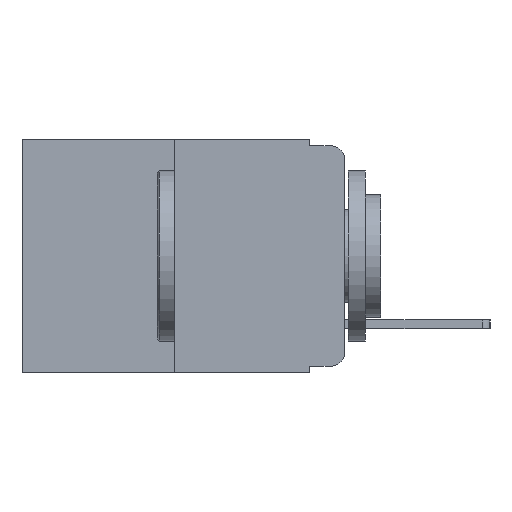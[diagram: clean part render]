
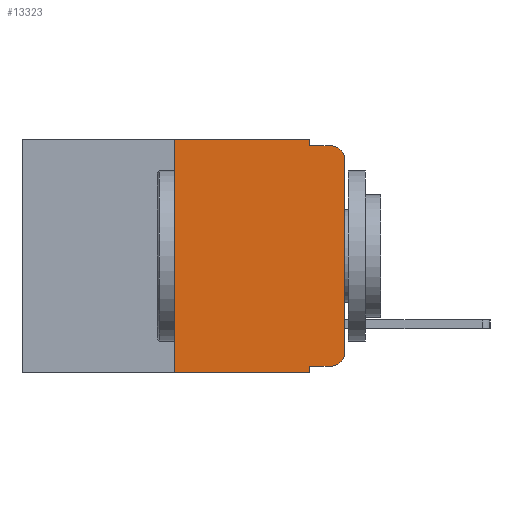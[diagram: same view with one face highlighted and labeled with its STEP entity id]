
A CAD part, left-side view. The second image highlights one B-rep face of the part: STEP entity #13323.
In plain terms, the highlighted planar face has unit normal (-1, 0, 0).
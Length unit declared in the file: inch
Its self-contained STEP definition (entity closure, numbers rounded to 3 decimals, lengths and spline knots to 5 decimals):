
#32 = VERTEX_POINT ( 'NONE', #4022 ) ;
#274 = EDGE_CURVE ( 'NONE', #12180, #11249, #820, .T. ) ;
#820 = CIRCLE ( 'NONE', #3981, 0.02 ) ;
#865 = DIRECTION ( 'NONE',  ( 0., 0., -1. ) ) ;
#1015 = DIRECTION ( 'NONE',  ( 0., 0., 1. ) ) ;
#1086 = CARTESIAN_POINT ( 'NONE',  ( 0., 0., -0.03 ) ) ;
#1105 = DIRECTION ( 'NONE',  ( 1., 0., 0. ) ) ;
#1246 = AXIS2_PLACEMENT_3D ( 'NONE', #20173, #1105, #12666 ) ;
#1468 = EDGE_CURVE ( 'NONE', #32, #12180, #20434, .T. ) ;
#1618 = VECTOR ( 'NONE', #16689, 39.37008 ) ;
#1734 = ORIENTED_EDGE ( 'NONE', *, *, #5015, .F. ) ;
#1923 = VERTEX_POINT ( 'NONE', #1086 ) ;
#2213 = FACE_OUTER_BOUND ( 'NONE', #7708, .T. ) ;
#3221 = LINE ( 'NONE', #3364, #11401 ) ;
#3364 = CARTESIAN_POINT ( 'NONE',  ( 0., 0.051, 0. ) ) ;
#3779 = CARTESIAN_POINT ( 'NONE',  ( 0., 0.051, -0.01 ) ) ;
#3981 = AXIS2_PLACEMENT_3D ( 'NONE', #9815, #9611, #9744 ) ;
#4022 = CARTESIAN_POINT ( 'NONE',  ( 0., 0.051, -0.333 ) ) ;
#4756 = ORIENTED_EDGE ( 'NONE', *, *, #9414, .F. ) ;
#4999 = CARTESIAN_POINT ( 'NONE',  ( 0., 0.02, -0.03 ) ) ;
#5015 = EDGE_CURVE ( 'NONE', #32, #10396, #14663, .T. ) ;
#5064 = DIRECTION ( 'NONE',  ( 0., 0., -1. ) ) ;
#5579 = VECTOR ( 'NONE', #7469, 39.37008 ) ;
#6145 = VERTEX_POINT ( 'NONE', #6284 ) ;
#6152 = EDGE_CURVE ( 'NONE', #7403, #9143, #10979, .T. ) ;
#6284 = CARTESIAN_POINT ( 'NONE',  ( 0., 0.02, -0.01 ) ) ;
#6298 = PLANE ( 'NONE',  #1246 ) ;
#6711 = DIRECTION ( 'NONE',  ( 0., 0., -1. ) ) ;
#7403 = VERTEX_POINT ( 'NONE', #14486 ) ;
#7469 = DIRECTION ( 'NONE',  ( 0., -1., 0. ) ) ;
#7708 = EDGE_LOOP ( 'NONE', ( #8176, #12787, #4756, #9636, #13758, #10147, #18208, #1734, #11089, #19154 ) ) ;
#8162 = CARTESIAN_POINT ( 'NONE',  ( 0., 0.051, -0.343 ) ) ;
#8176 = ORIENTED_EDGE ( 'NONE', *, *, #11510, .T. ) ;
#8318 = VECTOR ( 'NONE', #9204, 39.37008 ) ;
#8382 = EDGE_CURVE ( 'NONE', #11989, #13716, #3221, .T. ) ;
#9143 = VERTEX_POINT ( 'NONE', #10048 ) ;
#9204 = DIRECTION ( 'NONE',  ( 0., -1., 0. ) ) ;
#9414 = EDGE_CURVE ( 'NONE', #13716, #6145, #14488, .T. ) ;
#9477 = CARTESIAN_POINT ( 'NONE',  ( 0., 0., 0. ) ) ;
#9542 = CARTESIAN_POINT ( 'NONE',  ( 0., 0.25, 0. ) ) ;
#9611 = DIRECTION ( 'NONE',  ( -1., 0., 0. ) ) ;
#9636 = ORIENTED_EDGE ( 'NONE', *, *, #8382, .F. ) ;
#9744 = DIRECTION ( 'NONE',  ( 0., 0., -1. ) ) ;
#9815 = CARTESIAN_POINT ( 'NONE',  ( 0., 0.02, -0.313 ) ) ;
#10048 = CARTESIAN_POINT ( 'NONE',  ( 0., 0.25, 0. ) ) ;
#10147 = ORIENTED_EDGE ( 'NONE', *, *, #6152, .F. ) ;
#10396 = VERTEX_POINT ( 'NONE', #8162 ) ;
#10470 = EDGE_CURVE ( 'NONE', #1923, #6145, #10629, .T. ) ;
#10629 = CIRCLE ( 'NONE', #13852, 0.02 ) ;
#10979 = LINE ( 'NONE', #9542, #18570 ) ;
#11089 = ORIENTED_EDGE ( 'NONE', *, *, #1468, .T. ) ;
#11249 = VERTEX_POINT ( 'NONE', #18079 ) ;
#11401 = VECTOR ( 'NONE', #5064, 39.37008 ) ;
#11510 = EDGE_CURVE ( 'NONE', #11249, #1923, #15142, .T. ) ;
#11989 = VERTEX_POINT ( 'NONE', #12167 ) ;
#12167 = CARTESIAN_POINT ( 'NONE',  ( 0., 0.051, 0. ) ) ;
#12180 = VERTEX_POINT ( 'NONE', #12767 ) ;
#12609 = CARTESIAN_POINT ( 'NONE',  ( 0., 0.051, -0.333 ) ) ;
#12666 = DIRECTION ( 'NONE',  ( 0., 0., -1. ) ) ;
#12767 = CARTESIAN_POINT ( 'NONE',  ( 0., 0.02, -0.333 ) ) ;
#12787 = ORIENTED_EDGE ( 'NONE', *, *, #10470, .T. ) ;
#13252 = VECTOR ( 'NONE', #865, 39.37008 ) ;
#13323 = ADVANCED_FACE ( 'NONE', ( #2213 ), #6298, .F. ) ;
#13716 = VERTEX_POINT ( 'NONE', #3779 ) ;
#13758 = ORIENTED_EDGE ( 'NONE', *, *, #17898, .F. ) ;
#13844 = EDGE_CURVE ( 'NONE', #7403, #10396, #18593, .T. ) ;
#13852 = AXIS2_PLACEMENT_3D ( 'NONE', #4999, #16011, #6711 ) ;
#14486 = CARTESIAN_POINT ( 'NONE',  ( 0., 0.25, -0.343 ) ) ;
#14488 = LINE ( 'NONE', #15173, #5579 ) ;
#14663 = LINE ( 'NONE', #19980, #13252 ) ;
#15142 = LINE ( 'NONE', #9477, #19596 ) ;
#15173 = CARTESIAN_POINT ( 'NONE',  ( 0., 0.051, -0.01 ) ) ;
#15177 = CARTESIAN_POINT ( 'NONE',  ( 0., 0.473, -0.343 ) ) ;
#15230 = CARTESIAN_POINT ( 'NONE',  ( 0., 0.473, 0. ) ) ;
#16011 = DIRECTION ( 'NONE',  ( -1., 0., 0. ) ) ;
#16689 = DIRECTION ( 'NONE',  ( 0., -1., 0. ) ) ;
#16736 = DIRECTION ( 'NONE',  ( 0., -1., 0. ) ) ;
#17898 = EDGE_CURVE ( 'NONE', #9143, #11989, #19703, .T. ) ;
#18079 = CARTESIAN_POINT ( 'NONE',  ( 0., 0., -0.313 ) ) ;
#18208 = ORIENTED_EDGE ( 'NONE', *, *, #13844, .T. ) ;
#18570 = VECTOR ( 'NONE', #18653, 39.37008 ) ;
#18593 = LINE ( 'NONE', #15177, #1618 ) ;
#18653 = DIRECTION ( 'NONE',  ( 0., 0., 1. ) ) ;
#19154 = ORIENTED_EDGE ( 'NONE', *, *, #274, .T. ) ;
#19234 = VECTOR ( 'NONE', #16736, 39.37008 ) ;
#19596 = VECTOR ( 'NONE', #1015, 39.37008 ) ;
#19703 = LINE ( 'NONE', #15230, #19234 ) ;
#19980 = CARTESIAN_POINT ( 'NONE',  ( 0., 0.051, 0. ) ) ;
#20173 = CARTESIAN_POINT ( 'NONE',  ( 0., 0.473, 0. ) ) ;
#20434 = LINE ( 'NONE', #12609, #8318 ) ;
